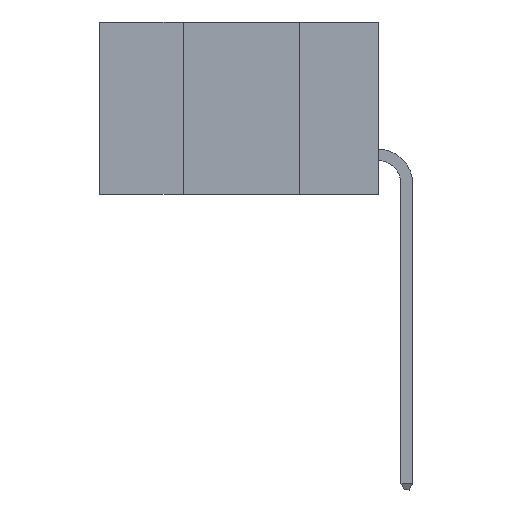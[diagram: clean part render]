
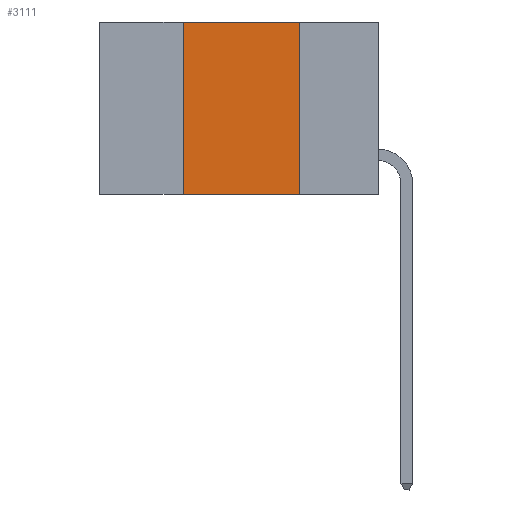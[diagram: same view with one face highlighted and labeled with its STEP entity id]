
A CAD part, left-side view. The second image highlights one B-rep face of the part: STEP entity #3111.
In plain terms, the highlighted planar face has unit normal (-1, 0, 0).
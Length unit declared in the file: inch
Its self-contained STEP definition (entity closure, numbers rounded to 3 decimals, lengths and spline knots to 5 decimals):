
#286 = VECTOR ( 'NONE', #8959, 39.37008 ) ;
#492 = EDGE_CURVE ( 'NONE', #1302, #4031, #8293, .T. ) ;
#811 = LINE ( 'NONE', #7683, #5355 ) ;
#892 = CARTESIAN_POINT ( 'NONE',  ( 0., 0.42, -0.37 ) ) ;
#1000 = DIRECTION ( 'NONE',  ( 0., 0., -1. ) ) ;
#1302 = VERTEX_POINT ( 'NONE', #892 ) ;
#1732 = DIRECTION ( 'NONE',  ( 0., -1., 0. ) ) ;
#2271 = VERTEX_POINT ( 'NONE', #6197 ) ;
#2569 = EDGE_LOOP ( 'NONE', ( #5287, #11685, #8489, #9946 ) ) ;
#2893 = CARTESIAN_POINT ( 'NONE',  ( 0., 0.17, 0. ) ) ;
#3066 = CARTESIAN_POINT ( 'NONE',  ( 0., 0.6, 0. ) ) ;
#3111 = ADVANCED_FACE ( 'NONE', ( #8941 ), #8568, .F. ) ;
#3873 = DIRECTION ( 'NONE',  ( 0., 0., 1. ) ) ;
#4031 = VERTEX_POINT ( 'NONE', #7185 ) ;
#4618 = CARTESIAN_POINT ( 'NONE',  ( 0., 0.6, 0. ) ) ;
#5287 = ORIENTED_EDGE ( 'NONE', *, *, #11163, .F. ) ;
#5355 = VECTOR ( 'NONE', #8584, 39.37008 ) ;
#5482 = CARTESIAN_POINT ( 'NONE',  ( 0., 0.6, -0.37 ) ) ;
#5543 = EDGE_CURVE ( 'NONE', #1302, #2271, #9673, .T. ) ;
#5891 = VECTOR ( 'NONE', #3873, 39.37008 ) ;
#6197 = CARTESIAN_POINT ( 'NONE',  ( 0., 0.17, -0.37 ) ) ;
#6398 = VERTEX_POINT ( 'NONE', #2893 ) ;
#7058 = VECTOR ( 'NONE', #1732, 39.37008 ) ;
#7185 = CARTESIAN_POINT ( 'NONE',  ( 0., 0.42, 0. ) ) ;
#7550 = AXIS2_PLACEMENT_3D ( 'NONE', #3066, #7620, #1000 ) ;
#7620 = DIRECTION ( 'NONE',  ( 1., 0., 0. ) ) ;
#7683 = CARTESIAN_POINT ( 'NONE',  ( 0., 0.17, 0. ) ) ;
#8293 = LINE ( 'NONE', #9412, #5891 ) ;
#8489 = ORIENTED_EDGE ( 'NONE', *, *, #492, .F. ) ;
#8568 = PLANE ( 'NONE',  #7550 ) ;
#8584 = DIRECTION ( 'NONE',  ( 0., 0., -1. ) ) ;
#8941 = FACE_OUTER_BOUND ( 'NONE', #2569, .T. ) ;
#8959 = DIRECTION ( 'NONE',  ( 0., -1., 0. ) ) ;
#9412 = CARTESIAN_POINT ( 'NONE',  ( 0., 0.42, 0. ) ) ;
#9456 = LINE ( 'NONE', #4618, #7058 ) ;
#9673 = LINE ( 'NONE', #5482, #286 ) ;
#9946 = ORIENTED_EDGE ( 'NONE', *, *, #5543, .T. ) ;
#11125 = EDGE_CURVE ( 'NONE', #4031, #6398, #9456, .T. ) ;
#11163 = EDGE_CURVE ( 'NONE', #6398, #2271, #811, .T. ) ;
#11685 = ORIENTED_EDGE ( 'NONE', *, *, #11125, .F. ) ;
